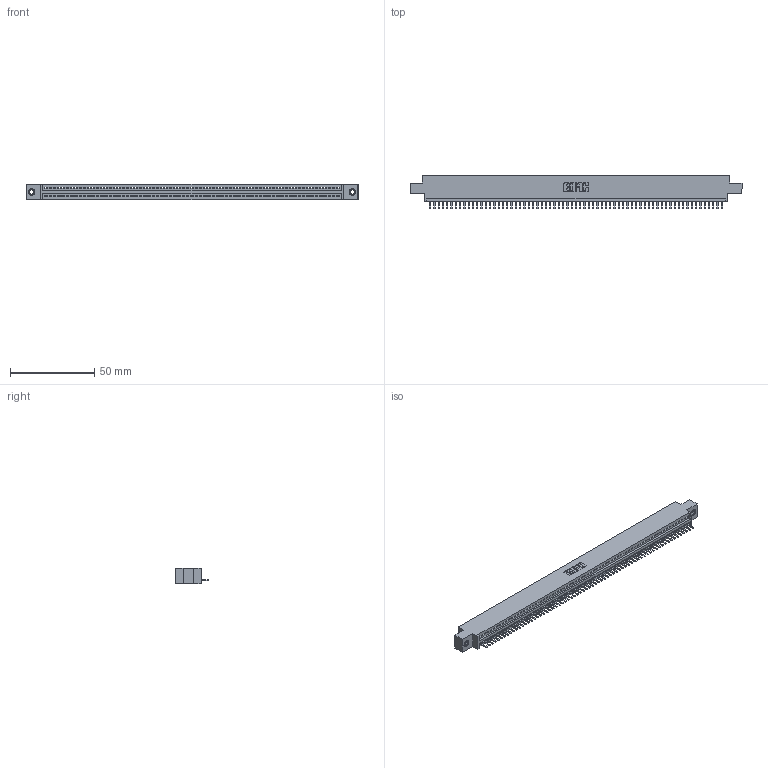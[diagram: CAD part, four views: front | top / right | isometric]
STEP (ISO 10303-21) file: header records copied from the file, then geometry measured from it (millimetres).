
FILE_DESCRIPTION (( 'STEP AP203' ), '1' );
FILE_NAME ('395-069-520-607.STEP', '2019-10-25T19:33:38', ( '' ), ( '' ), 'SwSTEP 2.0', 'SolidWorks 2016', '' );
FILE_SCHEMA (( 'CONFIG_CONTROL_DESIGN' ));
Length unit declared in the file: inch
Products named in the file (4): 345-292-001_345-293-120; 345 Part_0.170 Offset - 0.156 Dia-TI; 345-250-001_345-250-005-103; 395-069-520-607
Assembly tree (72 placements, depth 2):
  395-069-520-607
    345 Part_0.170 Offset - 0.156 Dia-TI
    345-292-001_345-293-120  x69
    345-250-001_345-250-005-103  x2
Bounding box: 196.47 x 19.68 x 9.4 mm (x, y, z)
Volume: 18556.6 mm3; surface area: 24536.8 mm2
Topology: 72 solids, 72 shells, 4468 faces, 13185 edges, 8598 vertices
Faces by surface type: plane 3014, cylinder 1438, cone 12, torus 4
Entity records: 49728 total; most frequent: CARTESIAN_POINT 8606, ORIENTED_EDGE 8590, DIRECTION 7491, EDGE_CURVE 4295, LINE 3863, VECTOR 3863, VERTEX_POINT 2856, AXIS2_PLACEMENT_3D 1814
